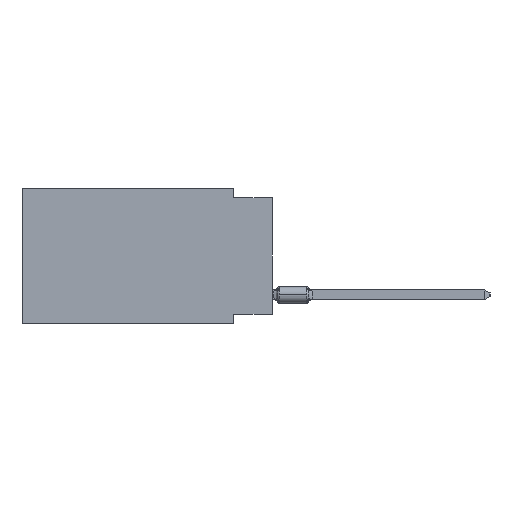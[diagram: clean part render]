
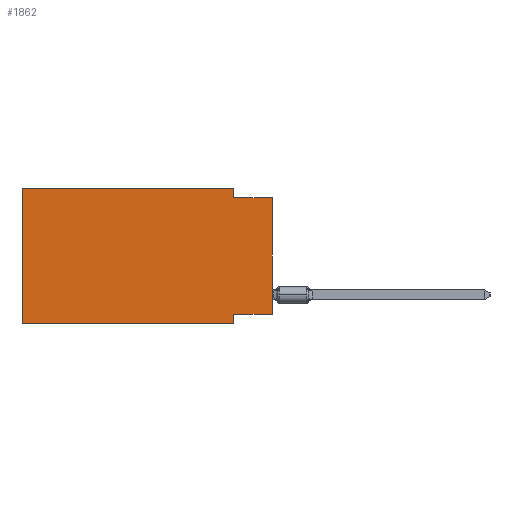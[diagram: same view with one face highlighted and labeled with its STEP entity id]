
A CAD part, left-side view. The second image highlights one B-rep face of the part: STEP entity #1862.
In plain terms, the highlighted planar face has unit normal (-1, 0, 0).
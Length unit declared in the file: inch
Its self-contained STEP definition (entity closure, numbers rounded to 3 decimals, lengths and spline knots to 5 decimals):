
#991 = VERTEX_POINT ( 'NONE', #14926 ) ;
#1627 = VERTEX_POINT ( 'NONE', #22526 ) ;
#1752 = LINE ( 'NONE', #7626, #11171 ) ;
#1862 = ADVANCED_FACE ( 'NONE', ( #23515 ), #8984, .F. ) ;
#2318 = ORIENTED_EDGE ( 'NONE', *, *, #5875, .F. ) ;
#3285 = EDGE_CURVE ( 'NONE', #14807, #991, #5920, .T. ) ;
#3636 = CARTESIAN_POINT ( 'NONE',  ( 0., 0.1, 0. ) ) ;
#3899 = EDGE_CURVE ( 'NONE', #21550, #3957, #24174, .T. ) ;
#3957 = VERTEX_POINT ( 'NONE', #9510 ) ;
#4049 = DIRECTION ( 'NONE',  ( 0., -1., 0. ) ) ;
#4798 = DIRECTION ( 'NONE',  ( 1., 0., 0. ) ) ;
#5314 = CARTESIAN_POINT ( 'NONE',  ( 0., 0., -0.325 ) ) ;
#5682 = DIRECTION ( 'NONE',  ( 0., 0., 1. ) ) ;
#5875 = EDGE_CURVE ( 'NONE', #991, #21550, #7257, .T. ) ;
#5920 = LINE ( 'NONE', #6049, #20324 ) ;
#6049 = CARTESIAN_POINT ( 'NONE',  ( 0., 0.645, 0. ) ) ;
#6114 = VECTOR ( 'NONE', #9073, 39.37008 ) ;
#7257 = LINE ( 'NONE', #22272, #14404 ) ;
#7276 = ORIENTED_EDGE ( 'NONE', *, *, #3899, .F. ) ;
#7387 = VECTOR ( 'NONE', #22340, 39.37008 ) ;
#7626 = CARTESIAN_POINT ( 'NONE',  ( 0., 0.645, -0.35 ) ) ;
#7662 = LINE ( 'NONE', #15179, #12390 ) ;
#7683 = EDGE_CURVE ( 'NONE', #3957, #22372, #10640, .T. ) ;
#8444 = ORIENTED_EDGE ( 'NONE', *, *, #22274, .T. ) ;
#8561 = ORIENTED_EDGE ( 'NONE', *, *, #7683, .F. ) ;
#8751 = LINE ( 'NONE', #5314, #10424 ) ;
#8766 = ORIENTED_EDGE ( 'NONE', *, *, #3285, .F. ) ;
#8984 = PLANE ( 'NONE',  #23589 ) ;
#9073 = DIRECTION ( 'NONE',  ( 0., 0., -1. ) ) ;
#9096 = CARTESIAN_POINT ( 'NONE',  ( 0., 0., -0.025 ) ) ;
#9510 = CARTESIAN_POINT ( 'NONE',  ( 0., 0.1, -0.025 ) ) ;
#10348 = DIRECTION ( 'NONE',  ( 0., 0., 1. ) ) ;
#10405 = CARTESIAN_POINT ( 'NONE',  ( 0., 0., -0.025 ) ) ;
#10424 = VECTOR ( 'NONE', #23764, 39.37008 ) ;
#10640 = LINE ( 'NONE', #10405, #20201 ) ;
#11171 = VECTOR ( 'NONE', #15139, 39.37008 ) ;
#11549 = CARTESIAN_POINT ( 'NONE',  ( 0., 0.1, -0.35 ) ) ;
#12390 = VECTOR ( 'NONE', #10348, 39.37008 ) ;
#13610 = EDGE_CURVE ( 'NONE', #1627, #22372, #7662, .T. ) ;
#14404 = VECTOR ( 'NONE', #4049, 39.37008 ) ;
#14807 = VERTEX_POINT ( 'NONE', #23953 ) ;
#14926 = CARTESIAN_POINT ( 'NONE',  ( 0., 0.645, 0. ) ) ;
#15139 = DIRECTION ( 'NONE',  ( 0., -1., 0. ) ) ;
#15179 = CARTESIAN_POINT ( 'NONE',  ( 0., 0., 0. ) ) ;
#15960 = EDGE_LOOP ( 'NONE', ( #19483, #8561, #7276, #2318, #8766, #8444, #17769, #23195 ) ) ;
#16488 = CARTESIAN_POINT ( 'NONE',  ( 0., 0.1, 0. ) ) ;
#16844 = CARTESIAN_POINT ( 'NONE',  ( 0., 0.1, -0.35 ) ) ;
#17769 = ORIENTED_EDGE ( 'NONE', *, *, #21486, .F. ) ;
#19483 = ORIENTED_EDGE ( 'NONE', *, *, #13610, .T. ) ;
#20043 = VERTEX_POINT ( 'NONE', #23519 ) ;
#20110 = DIRECTION ( 'NONE',  ( 0., -1., 0. ) ) ;
#20201 = VECTOR ( 'NONE', #20110, 39.37008 ) ;
#20292 = LINE ( 'NONE', #16844, #6114 ) ;
#20324 = VECTOR ( 'NONE', #5682, 39.37008 ) ;
#20413 = VERTEX_POINT ( 'NONE', #11549 ) ;
#21486 = EDGE_CURVE ( 'NONE', #20043, #20413, #20292, .T. ) ;
#21550 = VERTEX_POINT ( 'NONE', #16488 ) ;
#21915 = DIRECTION ( 'NONE',  ( 0., 0., -1. ) ) ;
#22147 = CARTESIAN_POINT ( 'NONE',  ( 0., 0.645, 0. ) ) ;
#22272 = CARTESIAN_POINT ( 'NONE',  ( 0., 0.645, 0. ) ) ;
#22274 = EDGE_CURVE ( 'NONE', #14807, #20413, #1752, .T. ) ;
#22340 = DIRECTION ( 'NONE',  ( 0., 0., -1. ) ) ;
#22372 = VERTEX_POINT ( 'NONE', #9096 ) ;
#22526 = CARTESIAN_POINT ( 'NONE',  ( 0., 0., -0.325 ) ) ;
#23195 = ORIENTED_EDGE ( 'NONE', *, *, #24027, .F. ) ;
#23515 = FACE_OUTER_BOUND ( 'NONE', #15960, .T. ) ;
#23519 = CARTESIAN_POINT ( 'NONE',  ( 0., 0.1, -0.325 ) ) ;
#23589 = AXIS2_PLACEMENT_3D ( 'NONE', #22147, #4798, #21915 ) ;
#23764 = DIRECTION ( 'NONE',  ( 0., 1., 0. ) ) ;
#23953 = CARTESIAN_POINT ( 'NONE',  ( 0., 0.645, -0.35 ) ) ;
#24027 = EDGE_CURVE ( 'NONE', #1627, #20043, #8751, .T. ) ;
#24174 = LINE ( 'NONE', #3636, #7387 ) ;
